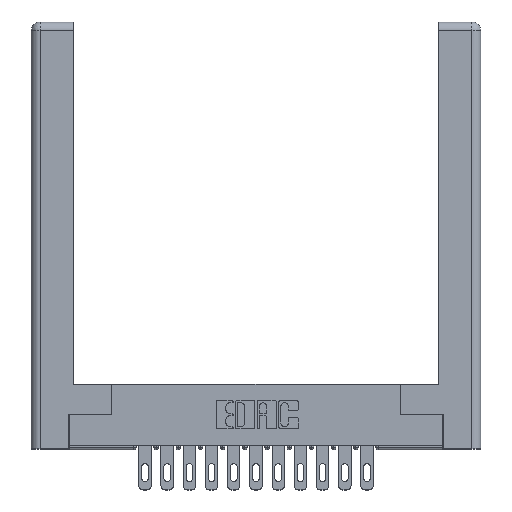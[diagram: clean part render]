
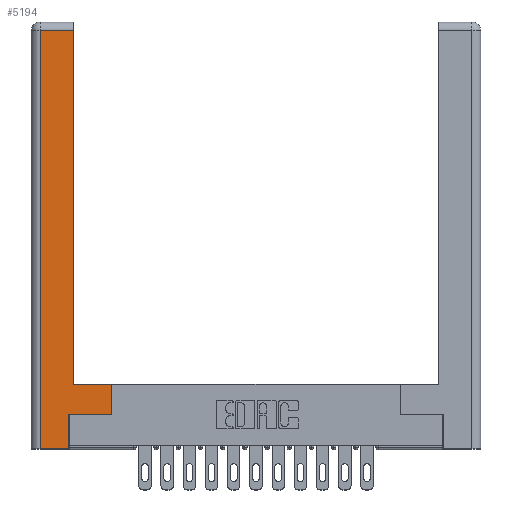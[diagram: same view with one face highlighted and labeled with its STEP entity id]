
A CAD part, top view. The second image highlights one B-rep face of the part: STEP entity #5194.
In plain terms, the highlighted planar face has unit normal (0, 0, 1).
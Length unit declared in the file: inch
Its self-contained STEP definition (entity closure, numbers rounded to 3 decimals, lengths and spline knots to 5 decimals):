
#94 = DIRECTION ( 'NONE',  ( 1., 0., 0. ) ) ;
#379 = VERTEX_POINT ( 'NONE', #8653 ) ;
#612 = CARTESIAN_POINT ( 'NONE',  ( 0.265, 0., 0. ) ) ;
#666 = CARTESIAN_POINT ( 'NONE',  ( 0.565, 0.45, 0. ) ) ;
#842 = LINE ( 'NONE', #8965, #5422 ) ;
#2140 = DIRECTION ( 'NONE',  ( -1., 0., 0. ) ) ;
#2181 = CARTESIAN_POINT ( 'NONE',  ( 0.295, 0.45, 0. ) ) ;
#2312 = DIRECTION ( 'NONE',  ( 0., 0., -1. ) ) ;
#2485 = VERTEX_POINT ( 'NONE', #666 ) ;
#2535 = ORIENTED_EDGE ( 'NONE', *, *, #6666, .T. ) ;
#2816 = LINE ( 'NONE', #13632, #14516 ) ;
#3045 = VERTEX_POINT ( 'NONE', #12745 ) ;
#3594 = VERTEX_POINT ( 'NONE', #5563 ) ;
#3963 = LINE ( 'NONE', #9259, #12101 ) ;
#4126 = EDGE_LOOP ( 'NONE', ( #8855, #2535, #17057, #9735, #16963, #8414, #10778, #10238 ) ) ;
#4252 = CARTESIAN_POINT ( 'NONE',  ( 0.0615, 2.94, 0. ) ) ;
#5194 = ADVANCED_FACE ( 'NONE', ( #8561 ), #6111, .F. ) ;
#5237 = DIRECTION ( 'NONE',  ( 0., 1., 0. ) ) ;
#5422 = VECTOR ( 'NONE', #15456, 39.37008 ) ;
#5563 = CARTESIAN_POINT ( 'NONE',  ( 0.565, 0.245, 0. ) ) ;
#5655 = VECTOR ( 'NONE', #5237, 39.37008 ) ;
#6111 = PLANE ( 'NONE',  #13211 ) ;
#6494 = VECTOR ( 'NONE', #2140, 39.37008 ) ;
#6506 = EDGE_CURVE ( 'NONE', #10694, #16622, #13127, .T. ) ;
#6638 = CARTESIAN_POINT ( 'NONE',  ( 0.265, 0.245, 0. ) ) ;
#6647 = EDGE_CURVE ( 'NONE', #10945, #379, #9230, .T. ) ;
#6666 = EDGE_CURVE ( 'NONE', #379, #7060, #2816, .T. ) ;
#7060 = VERTEX_POINT ( 'NONE', #4252 ) ;
#7801 = LINE ( 'NONE', #11879, #10162 ) ;
#8050 = EDGE_CURVE ( 'NONE', #3594, #2485, #842, .T. ) ;
#8414 = ORIENTED_EDGE ( 'NONE', *, *, #8708, .T. ) ;
#8561 = FACE_OUTER_BOUND ( 'NONE', #4126, .T. ) ;
#8628 = LINE ( 'NONE', #12607, #6494 ) ;
#8653 = CARTESIAN_POINT ( 'NONE',  ( 0.295, 2.94, 0. ) ) ;
#8708 = EDGE_CURVE ( 'NONE', #16622, #3594, #7801, .T. ) ;
#8855 = ORIENTED_EDGE ( 'NONE', *, *, #6647, .T. ) ;
#8965 = CARTESIAN_POINT ( 'NONE',  ( 0.565, 0.45, 0. ) ) ;
#9094 = CARTESIAN_POINT ( 'NONE',  ( 0.0615, 0., 0. ) ) ;
#9198 = EDGE_CURVE ( 'NONE', #7060, #3045, #9254, .T. ) ;
#9230 = LINE ( 'NONE', #13305, #5655 ) ;
#9254 = LINE ( 'NONE', #9094, #17077 ) ;
#9259 = CARTESIAN_POINT ( 'NONE',  ( 0.265, 0., 0. ) ) ;
#9735 = ORIENTED_EDGE ( 'NONE', *, *, #10457, .T. ) ;
#10162 = VECTOR ( 'NONE', #13086, 39.37008 ) ;
#10238 = ORIENTED_EDGE ( 'NONE', *, *, #12991, .T. ) ;
#10457 = EDGE_CURVE ( 'NONE', #3045, #10694, #3963, .T. ) ;
#10694 = VERTEX_POINT ( 'NONE', #612 ) ;
#10778 = ORIENTED_EDGE ( 'NONE', *, *, #8050, .T. ) ;
#10785 = DIRECTION ( 'NONE',  ( -1., 0., 0. ) ) ;
#10945 = VERTEX_POINT ( 'NONE', #2181 ) ;
#11737 = DIRECTION ( 'NONE',  ( 0., 1., 0. ) ) ;
#11879 = CARTESIAN_POINT ( 'NONE',  ( 0.565, 0.245, 0. ) ) ;
#12101 = VECTOR ( 'NONE', #94, 39.37008 ) ;
#12530 = DIRECTION ( 'NONE',  ( -1., 0., 0. ) ) ;
#12607 = CARTESIAN_POINT ( 'NONE',  ( 0.295, 0.45, 0. ) ) ;
#12713 = CARTESIAN_POINT ( 'NONE',  ( 0., 0., 0. ) ) ;
#12745 = CARTESIAN_POINT ( 'NONE',  ( 0.0615, 0., 0. ) ) ;
#12991 = EDGE_CURVE ( 'NONE', #2485, #10945, #8628, .T. ) ;
#13086 = DIRECTION ( 'NONE',  ( 1., 0., 0. ) ) ;
#13127 = LINE ( 'NONE', #6638, #15621 ) ;
#13211 = AXIS2_PLACEMENT_3D ( 'NONE', #12713, #2312, #12530 ) ;
#13305 = CARTESIAN_POINT ( 'NONE',  ( 0.295, 3., 0. ) ) ;
#13632 = CARTESIAN_POINT ( 'NONE',  ( 0.0615, 2.94, 0. ) ) ;
#14463 = CARTESIAN_POINT ( 'NONE',  ( 0.265, 0.245, 0. ) ) ;
#14516 = VECTOR ( 'NONE', #10785, 39.37008 ) ;
#14531 = DIRECTION ( 'NONE',  ( 0., -1., 0. ) ) ;
#15456 = DIRECTION ( 'NONE',  ( 0., 1., 0. ) ) ;
#15621 = VECTOR ( 'NONE', #11737, 39.37008 ) ;
#16622 = VERTEX_POINT ( 'NONE', #14463 ) ;
#16963 = ORIENTED_EDGE ( 'NONE', *, *, #6506, .T. ) ;
#17057 = ORIENTED_EDGE ( 'NONE', *, *, #9198, .T. ) ;
#17077 = VECTOR ( 'NONE', #14531, 39.37008 ) ;
